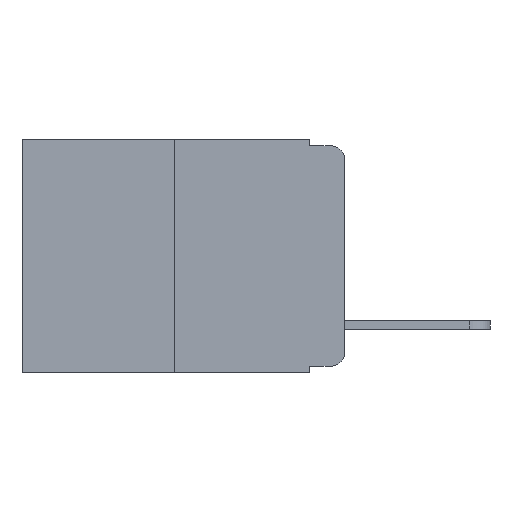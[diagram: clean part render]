
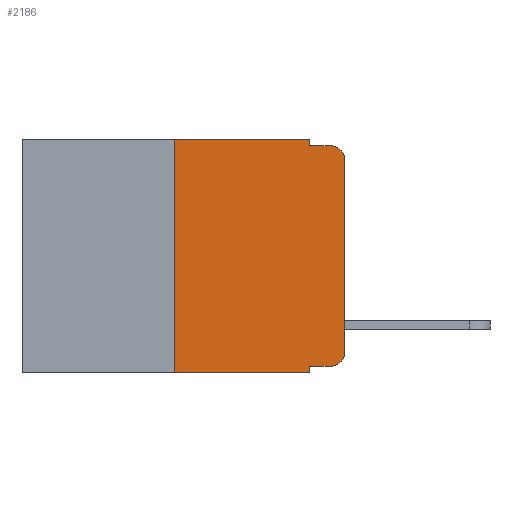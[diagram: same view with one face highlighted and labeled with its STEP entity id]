
A CAD part, left-side view. The second image highlights one B-rep face of the part: STEP entity #2186.
In plain terms, the highlighted planar face has unit normal (-1, 0, 0).
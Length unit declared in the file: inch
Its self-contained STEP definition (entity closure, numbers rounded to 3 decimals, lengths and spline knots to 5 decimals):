
#129 = CARTESIAN_POINT ( 'NONE',  ( 0., 0.051, -0.01 ) ) ;
#217 = DIRECTION ( 'NONE',  ( -1., 0., 0. ) ) ;
#447 = ORIENTED_EDGE ( 'NONE', *, *, #20785, .F. ) ;
#768 = ORIENTED_EDGE ( 'NONE', *, *, #16557, .F. ) ;
#856 = ORIENTED_EDGE ( 'NONE', *, *, #9355, .T. ) ;
#1083 = CARTESIAN_POINT ( 'NONE',  ( 0., 0., -0.03 ) ) ;
#1154 = VERTEX_POINT ( 'NONE', #6778 ) ;
#1314 = AXIS2_PLACEMENT_3D ( 'NONE', #15227, #6421, #18740 ) ;
#2004 = VERTEX_POINT ( 'NONE', #2622 ) ;
#2133 = VERTEX_POINT ( 'NONE', #2853 ) ;
#2186 = ADVANCED_FACE ( 'NONE', ( #7752 ), #4476, .F. ) ;
#2337 = LINE ( 'NONE', #6196, #9275 ) ;
#2558 = VECTOR ( 'NONE', #13482, 39.37008 ) ;
#2622 = CARTESIAN_POINT ( 'NONE',  ( 0., 0., -0.313 ) ) ;
#2678 = VECTOR ( 'NONE', #16234, 39.37008 ) ;
#2747 = CARTESIAN_POINT ( 'NONE',  ( 0., 0.473, 0. ) ) ;
#2853 = CARTESIAN_POINT ( 'NONE',  ( 0., 0.02, -0.01 ) ) ;
#2873 = CARTESIAN_POINT ( 'NONE',  ( 0., 0.02, -0.333 ) ) ;
#2883 = ORIENTED_EDGE ( 'NONE', *, *, #5995, .F. ) ;
#3334 = LINE ( 'NONE', #22801, #19616 ) ;
#3945 = CARTESIAN_POINT ( 'NONE',  ( 0., 0.051, -0.333 ) ) ;
#4476 = PLANE ( 'NONE',  #1314 ) ;
#4964 = VERTEX_POINT ( 'NONE', #17264 ) ;
#5034 = ORIENTED_EDGE ( 'NONE', *, *, #7214, .T. ) ;
#5070 = VERTEX_POINT ( 'NONE', #17660 ) ;
#5256 = EDGE_CURVE ( 'NONE', #16543, #5070, #7589, .T. ) ;
#5281 = LINE ( 'NONE', #21487, #19902 ) ;
#5798 = CARTESIAN_POINT ( 'NONE',  ( 0., 0., 0. ) ) ;
#5995 = EDGE_CURVE ( 'NONE', #19344, #15355, #13367, .T. ) ;
#6008 = VERTEX_POINT ( 'NONE', #1083 ) ;
#6108 = LINE ( 'NONE', #2747, #8322 ) ;
#6196 = CARTESIAN_POINT ( 'NONE',  ( 0., 0.473, -0.343 ) ) ;
#6206 = CARTESIAN_POINT ( 'NONE',  ( 0., 0.051, 0. ) ) ;
#6421 = DIRECTION ( 'NONE',  ( 1., 0., 0. ) ) ;
#6470 = ORIENTED_EDGE ( 'NONE', *, *, #20439, .T. ) ;
#6778 = CARTESIAN_POINT ( 'NONE',  ( 0., 0.25, 0. ) ) ;
#6923 = EDGE_CURVE ( 'NONE', #16543, #18164, #5281, .T. ) ;
#7214 = EDGE_CURVE ( 'NONE', #18164, #2004, #11354, .T. ) ;
#7589 = LINE ( 'NONE', #10247, #18328 ) ;
#7752 = FACE_OUTER_BOUND ( 'NONE', #15734, .T. ) ;
#8322 = VECTOR ( 'NONE', #16850, 39.37008 ) ;
#9095 = DIRECTION ( 'NONE',  ( 0., -1., 0. ) ) ;
#9142 = DIRECTION ( 'NONE',  ( 0., 0., 1. ) ) ;
#9172 = DIRECTION ( 'NONE',  ( 0., 0., -1. ) ) ;
#9195 = DIRECTION ( 'NONE',  ( 0., 0., -1. ) ) ;
#9275 = VECTOR ( 'NONE', #18672, 39.37008 ) ;
#9355 = EDGE_CURVE ( 'NONE', #2004, #6008, #12091, .T. ) ;
#9718 = CIRCLE ( 'NONE', #17541, 0.02 ) ;
#10247 = CARTESIAN_POINT ( 'NONE',  ( 0., 0.051, 0. ) ) ;
#11354 = CIRCLE ( 'NONE', #14267, 0.02 ) ;
#11792 = DIRECTION ( 'NONE',  ( 0., 0., -1. ) ) ;
#12091 = LINE ( 'NONE', #5798, #2678 ) ;
#12436 = EDGE_CURVE ( 'NONE', #4964, #5070, #2337, .T. ) ;
#12509 = CARTESIAN_POINT ( 'NONE',  ( 0., 0.02, -0.03 ) ) ;
#13367 = LINE ( 'NONE', #6206, #2558 ) ;
#13482 = DIRECTION ( 'NONE',  ( 0., 0., -1. ) ) ;
#14195 = DIRECTION ( 'NONE',  ( -1., 0., 0. ) ) ;
#14267 = AXIS2_PLACEMENT_3D ( 'NONE', #22861, #14195, #9172 ) ;
#14577 = ORIENTED_EDGE ( 'NONE', *, *, #16906, .F. ) ;
#15142 = LINE ( 'NONE', #21758, #22005 ) ;
#15227 = CARTESIAN_POINT ( 'NONE',  ( 0., 0.473, 0. ) ) ;
#15355 = VERTEX_POINT ( 'NONE', #129 ) ;
#15734 = EDGE_LOOP ( 'NONE', ( #856, #6470, #14577, #2883, #447, #768, #16463, #19179, #16404, #5034 ) ) ;
#16234 = DIRECTION ( 'NONE',  ( 0., 0., 1. ) ) ;
#16404 = ORIENTED_EDGE ( 'NONE', *, *, #6923, .T. ) ;
#16463 = ORIENTED_EDGE ( 'NONE', *, *, #12436, .T. ) ;
#16543 = VERTEX_POINT ( 'NONE', #3945 ) ;
#16557 = EDGE_CURVE ( 'NONE', #4964, #1154, #15142, .T. ) ;
#16850 = DIRECTION ( 'NONE',  ( 0., -1., 0. ) ) ;
#16906 = EDGE_CURVE ( 'NONE', #15355, #2133, #3334, .T. ) ;
#17264 = CARTESIAN_POINT ( 'NONE',  ( 0., 0.25, -0.343 ) ) ;
#17541 = AXIS2_PLACEMENT_3D ( 'NONE', #12509, #217, #9195 ) ;
#17660 = CARTESIAN_POINT ( 'NONE',  ( 0., 0.051, -0.343 ) ) ;
#18164 = VERTEX_POINT ( 'NONE', #2873 ) ;
#18328 = VECTOR ( 'NONE', #11792, 39.37008 ) ;
#18672 = DIRECTION ( 'NONE',  ( 0., -1., 0. ) ) ;
#18740 = DIRECTION ( 'NONE',  ( 0., 0., -1. ) ) ;
#18785 = CARTESIAN_POINT ( 'NONE',  ( 0., 0.051, 0. ) ) ;
#19179 = ORIENTED_EDGE ( 'NONE', *, *, #5256, .F. ) ;
#19344 = VERTEX_POINT ( 'NONE', #18785 ) ;
#19616 = VECTOR ( 'NONE', #22719, 39.37008 ) ;
#19902 = VECTOR ( 'NONE', #9095, 39.37008 ) ;
#20439 = EDGE_CURVE ( 'NONE', #6008, #2133, #9718, .T. ) ;
#20785 = EDGE_CURVE ( 'NONE', #1154, #19344, #6108, .T. ) ;
#21487 = CARTESIAN_POINT ( 'NONE',  ( 0., 0.051, -0.333 ) ) ;
#21758 = CARTESIAN_POINT ( 'NONE',  ( 0., 0.25, 0. ) ) ;
#22005 = VECTOR ( 'NONE', #9142, 39.37008 ) ;
#22719 = DIRECTION ( 'NONE',  ( 0., -1., 0. ) ) ;
#22801 = CARTESIAN_POINT ( 'NONE',  ( 0., 0.051, -0.01 ) ) ;
#22861 = CARTESIAN_POINT ( 'NONE',  ( 0., 0.02, -0.313 ) ) ;
